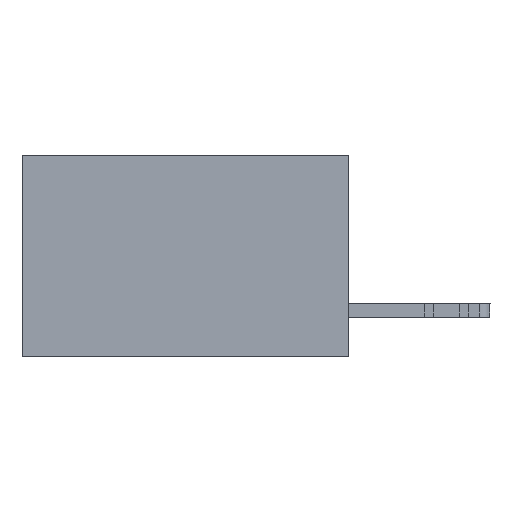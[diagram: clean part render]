
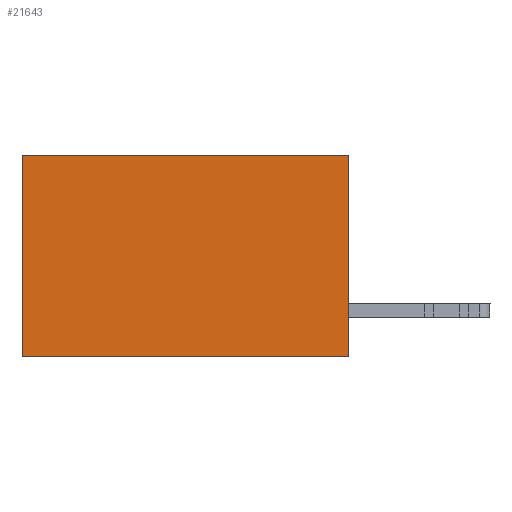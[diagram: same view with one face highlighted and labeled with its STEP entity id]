
A CAD part, left-side view. The second image highlights one B-rep face of the part: STEP entity #21643.
In plain terms, the highlighted planar face has unit normal (-1, 0, 0).
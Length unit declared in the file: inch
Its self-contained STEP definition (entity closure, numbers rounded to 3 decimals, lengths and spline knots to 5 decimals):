
#492 = CARTESIAN_POINT ( 'NONE',  ( 0.2615, 0., 0. ) ) ;
#2061 = LINE ( 'NONE', #9317, #17126 ) ;
#2166 = LINE ( 'NONE', #22357, #22959 ) ;
#3341 = DIRECTION ( 'NONE',  ( 0., 0., -1. ) ) ;
#3566 = AXIS2_PLACEMENT_3D ( 'NONE', #20510, #8943, #22461 ) ;
#3666 = EDGE_CURVE ( 'NONE', #10870, #24627, #13058, .T. ) ;
#3743 = VECTOR ( 'NONE', #14083, 39.37008 ) ;
#4323 = EDGE_CURVE ( 'NONE', #4693, #13996, #2166, .T. ) ;
#4693 = VERTEX_POINT ( 'NONE', #492 ) ;
#6255 = ORIENTED_EDGE ( 'NONE', *, *, #14128, .F. ) ;
#6917 = PLANE ( 'NONE',  #3566 ) ;
#8943 = DIRECTION ( 'NONE',  ( 1., 0., 0. ) ) ;
#9317 = CARTESIAN_POINT ( 'NONE',  ( 0.2615, 0., -0.37 ) ) ;
#10700 = DIRECTION ( 'NONE',  ( 0., 1., 0. ) ) ;
#10870 = VERTEX_POINT ( 'NONE', #16735 ) ;
#11522 = FACE_OUTER_BOUND ( 'NONE', #12246, .T. ) ;
#12246 = EDGE_LOOP ( 'NONE', ( #12534, #22915, #6255, #21225 ) ) ;
#12510 = CARTESIAN_POINT ( 'NONE',  ( 0.2615, 0.6, -0.37 ) ) ;
#12534 = ORIENTED_EDGE ( 'NONE', *, *, #16743, .T. ) ;
#12819 = CARTESIAN_POINT ( 'NONE',  ( 0.2615, 0.6, 0. ) ) ;
#13058 = LINE ( 'NONE', #13739, #3743 ) ;
#13739 = CARTESIAN_POINT ( 'NONE',  ( 0.2615, 0., -0.37 ) ) ;
#13996 = VERTEX_POINT ( 'NONE', #12819 ) ;
#14083 = DIRECTION ( 'NONE',  ( 0., 1., 0. ) ) ;
#14128 = EDGE_CURVE ( 'NONE', #4693, #10870, #2061, .T. ) ;
#14366 = LINE ( 'NONE', #21159, #17189 ) ;
#16735 = CARTESIAN_POINT ( 'NONE',  ( 0.2615, 0., -0.37 ) ) ;
#16743 = EDGE_CURVE ( 'NONE', #13996, #24627, #14366, .T. ) ;
#17126 = VECTOR ( 'NONE', #3341, 39.37008 ) ;
#17189 = VECTOR ( 'NONE', #17287, 39.37008 ) ;
#17287 = DIRECTION ( 'NONE',  ( 0., 0., -1. ) ) ;
#20510 = CARTESIAN_POINT ( 'NONE',  ( 0.2615, 0., -0.37 ) ) ;
#21159 = CARTESIAN_POINT ( 'NONE',  ( 0.2615, 0.6, -0.37 ) ) ;
#21225 = ORIENTED_EDGE ( 'NONE', *, *, #4323, .T. ) ;
#21643 = ADVANCED_FACE ( 'NONE', ( #11522 ), #6917, .F. ) ;
#22357 = CARTESIAN_POINT ( 'NONE',  ( 0.2615, 0., 0. ) ) ;
#22461 = DIRECTION ( 'NONE',  ( 0., 0., -1. ) ) ;
#22915 = ORIENTED_EDGE ( 'NONE', *, *, #3666, .F. ) ;
#22959 = VECTOR ( 'NONE', #10700, 39.37008 ) ;
#24627 = VERTEX_POINT ( 'NONE', #12510 ) ;
